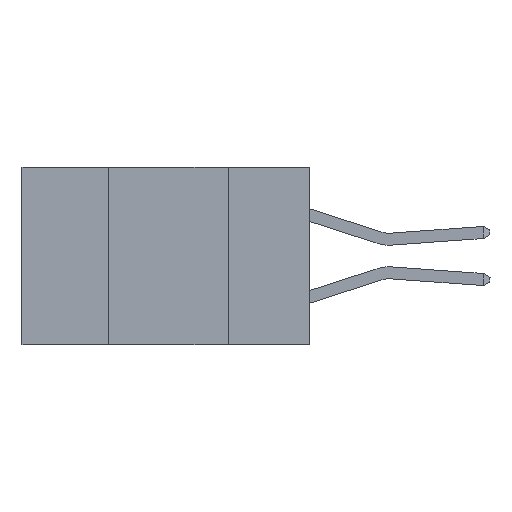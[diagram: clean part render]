
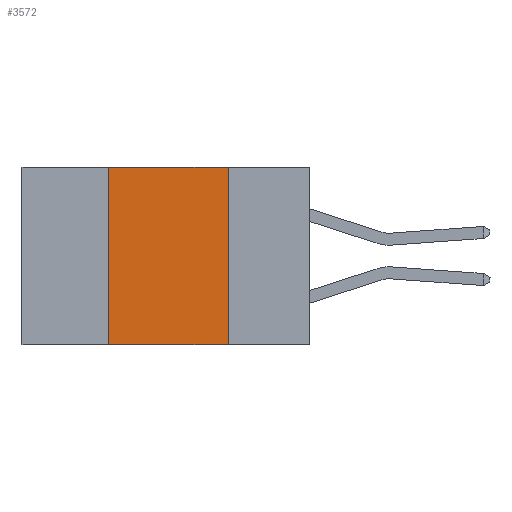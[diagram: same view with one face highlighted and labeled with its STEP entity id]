
A CAD part, left-side view. The second image highlights one B-rep face of the part: STEP entity #3572.
In plain terms, the highlighted planar face has unit normal (-1, 0, 0).
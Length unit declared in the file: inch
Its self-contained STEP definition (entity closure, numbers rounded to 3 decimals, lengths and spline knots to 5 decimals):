
#314 = DIRECTION ( 'NONE',  ( 0., 0., -1. ) ) ;
#568 = CARTESIAN_POINT ( 'NONE',  ( 0., 0.6, 0. ) ) ;
#679 = VECTOR ( 'NONE', #9725, 39.37008 ) ;
#1732 = VERTEX_POINT ( 'NONE', #6148 ) ;
#1830 = FACE_OUTER_BOUND ( 'NONE', #10196, .T. ) ;
#1884 = CARTESIAN_POINT ( 'NONE',  ( 0., 0.17, 0. ) ) ;
#1926 = ORIENTED_EDGE ( 'NONE', *, *, #8723, .F. ) ;
#2263 = VECTOR ( 'NONE', #314, 39.37008 ) ;
#2507 = LINE ( 'NONE', #3065, #4590 ) ;
#2552 = EDGE_CURVE ( 'NONE', #3319, #2783, #2781, .T. ) ;
#2571 = DIRECTION ( 'NONE',  ( 0., 0., -1. ) ) ;
#2781 = LINE ( 'NONE', #9510, #679 ) ;
#2783 = VERTEX_POINT ( 'NONE', #3062 ) ;
#3062 = CARTESIAN_POINT ( 'NONE',  ( 0., 0.42, 0. ) ) ;
#3065 = CARTESIAN_POINT ( 'NONE',  ( 0., 0.6, -0.37 ) ) ;
#3319 = VERTEX_POINT ( 'NONE', #5816 ) ;
#3360 = CARTESIAN_POINT ( 'NONE',  ( 0., 0.17, 0. ) ) ;
#3572 = ADVANCED_FACE ( 'NONE', ( #1830 ), #4207, .F. ) ;
#4207 = PLANE ( 'NONE',  #8505 ) ;
#4590 = VECTOR ( 'NONE', #6363, 39.37008 ) ;
#4978 = EDGE_CURVE ( 'NONE', #3319, #1732, #2507, .T. ) ;
#5238 = ORIENTED_EDGE ( 'NONE', *, *, #7102, .F. ) ;
#5816 = CARTESIAN_POINT ( 'NONE',  ( 0., 0.42, -0.37 ) ) ;
#6148 = CARTESIAN_POINT ( 'NONE',  ( 0., 0.17, -0.37 ) ) ;
#6363 = DIRECTION ( 'NONE',  ( 0., -1., 0. ) ) ;
#6457 = DIRECTION ( 'NONE',  ( 0., -1., 0. ) ) ;
#6658 = LINE ( 'NONE', #568, #6918 ) ;
#6715 = LINE ( 'NONE', #1884, #2263 ) ;
#6744 = DIRECTION ( 'NONE',  ( 1., 0., 0. ) ) ;
#6918 = VECTOR ( 'NONE', #6457, 39.37008 ) ;
#7102 = EDGE_CURVE ( 'NONE', #9559, #1732, #6715, .T. ) ;
#8499 = ORIENTED_EDGE ( 'NONE', *, *, #2552, .F. ) ;
#8505 = AXIS2_PLACEMENT_3D ( 'NONE', #10058, #6744, #2571 ) ;
#8723 = EDGE_CURVE ( 'NONE', #2783, #9559, #6658, .T. ) ;
#8991 = ORIENTED_EDGE ( 'NONE', *, *, #4978, .T. ) ;
#9510 = CARTESIAN_POINT ( 'NONE',  ( 0., 0.42, 0. ) ) ;
#9559 = VERTEX_POINT ( 'NONE', #3360 ) ;
#9725 = DIRECTION ( 'NONE',  ( 0., 0., 1. ) ) ;
#10058 = CARTESIAN_POINT ( 'NONE',  ( 0., 0.6, 0. ) ) ;
#10196 = EDGE_LOOP ( 'NONE', ( #5238, #1926, #8499, #8991 ) ) ;
